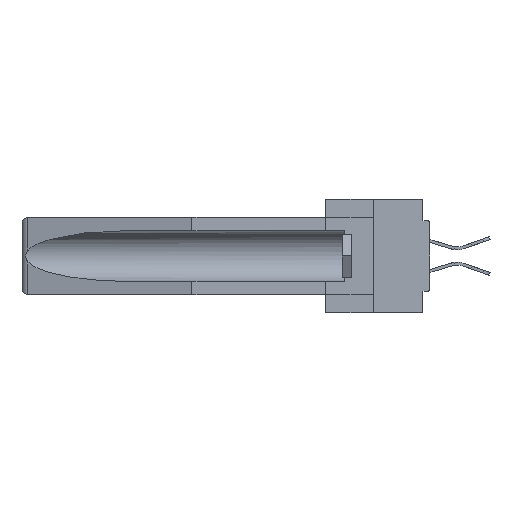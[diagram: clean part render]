
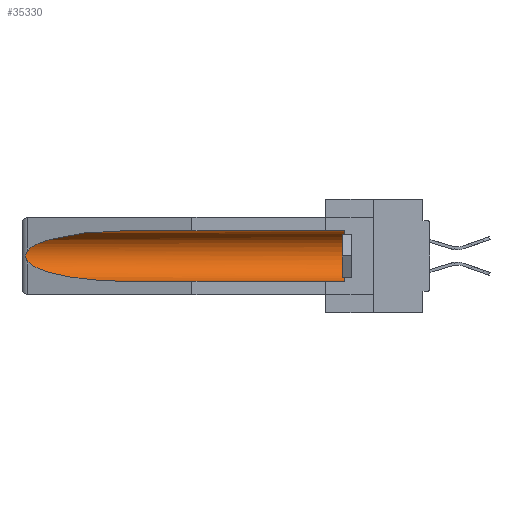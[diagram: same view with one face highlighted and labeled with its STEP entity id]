
A CAD part, left-side view. The second image highlights one B-rep face of the part: STEP entity #35330.
In plain terms, the highlighted cylindrical face has radius 2.857 mm (diameter 5.715 mm), a partial arc.
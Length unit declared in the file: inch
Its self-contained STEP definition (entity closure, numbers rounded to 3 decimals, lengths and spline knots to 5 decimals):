
#68 = DIRECTION ( 'NONE',  ( 0., 0., 1. ) ) ;
#99 = DIRECTION ( 'NONE',  ( 0., 0., 1. ) ) ;
#173 = CARTESIAN_POINT ( 'NONE',  ( 0.2673, 1.5327, -0.16383 ) ) ;
#321 = CARTESIAN_POINT ( 'NONE',  ( 0.2673, 1.53269, -0.17917 ) ) ;
#473 = CARTESIAN_POINT ( 'NONE',  ( 0.26654, 1.53092, -0.15636 ) ) ;
#629 = CARTESIAN_POINT ( 'NONE',  ( 0.26597, 1.5296, -0.19026 ) ) ;
#797 = LINE ( 'NONE', #43231, #3456 ) ;
#1778 = CARTESIAN_POINT ( 'NONE',  ( 0.26537, 1.52718, -0.19328 ) ) ;
#2358 = CARTESIAN_POINT ( 'NONE',  ( 0.21114, 1.30732, -0.284 ) ) ;
#3456 = VECTOR ( 'NONE', #29276, 39.37008 ) ;
#4014 = EDGE_CURVE ( 'NONE', #23667, #7533, #10403, .T. ) ;
#5608 = CARTESIAN_POINT ( 'NONE',  ( 0.155, 1.07973, -0.059 ) ) ;
#6609 = ORIENTED_EDGE ( 'NONE', *, *, #7077, .F. ) ;
#7077 = EDGE_CURVE ( 'NONE', #41100, #7533, #18135, .T. ) ;
#7160 = CARTESIAN_POINT ( 'NONE',  ( 0.26537, 1.52718, -0.19328 ) ) ;
#7533 = VERTEX_POINT ( 'NONE', #36277 ) ;
#10403 =( BOUNDED_CURVE ( )  B_SPLINE_CURVE ( 3, ( #1778, #12531, #2358, #19693 ),
 .UNSPECIFIED., .F., .F. ) 
 B_SPLINE_CURVE_WITH_KNOTS ( ( 4, 4 ),
 ( 0.1948, 1.5708 ),
 .UNSPECIFIED. ) 
 CURVE ( )  GEOMETRIC_REPRESENTATION_ITEM ( )  RATIONAL_B_SPLINE_CURVE ( ( 1., 0.848, 0.848, 1. ) ) 
 REPRESENTATION_ITEM ( '' )  );
#11840 = CARTESIAN_POINT ( 'NONE',  ( 0.155, 0.126, -0.059 ) ) ;
#12379 = ORIENTED_EDGE ( 'NONE', *, *, #4014, .T. ) ;
#12434 = CARTESIAN_POINT ( 'NONE',  ( 0.26537, 1.52718, -0.14972 ) ) ;
#12531 = CARTESIAN_POINT ( 'NONE',  ( 0.25451, 1.48313, -0.24835 ) ) ;
#13896 = DIRECTION ( 'NONE',  ( 0., -1., 0. ) ) ;
#13972 = CARTESIAN_POINT ( 'NONE',  ( 0.26537, 1.52718, -0.14972 ) ) ;
#13990 = CYLINDRICAL_SURFACE ( 'NONE', #24446, 0.1125 ) ;
#15562 = VERTEX_POINT ( 'NONE', #11840 ) ;
#15887 = VERTEX_POINT ( 'NONE', #28764 ) ;
#17029 = VECTOR ( 'NONE', #18907, 39.37008 ) ;
#17481 = CARTESIAN_POINT ( 'NONE',  ( 0.26597, 1.52961, -0.15275 ) ) ;
#17610 = ORIENTED_EDGE ( 'NONE', *, *, #39559, .T. ) ;
#17627 = CARTESIAN_POINT ( 'NONE',  ( 0.26655, 1.53094, -0.18657 ) ) ;
#18135 = LINE ( 'NONE', #43104, #17029 ) ;
#18243 = EDGE_CURVE ( 'NONE', #15887, #23667, #23204, .T. ) ;
#18907 = DIRECTION ( 'NONE',  ( 0., 1., 0. ) ) ;
#19693 = CARTESIAN_POINT ( 'NONE',  ( 0.155, 1.07973, -0.284 ) ) ;
#20891 = CARTESIAN_POINT ( 'NONE',  ( 0.155, 0.126, -0.1715 ) ) ;
#21831 = CARTESIAN_POINT ( 'NONE',  ( 0.26537, 1.52718, -0.19328 ) ) ;
#23025 = ORIENTED_EDGE ( 'NONE', *, *, #25254, .T. ) ;
#23195 = EDGE_LOOP ( 'NONE', ( #23025, #41322, #12379, #6609, #17610, #30607 ) ) ;
#23204 = B_SPLINE_CURVE_WITH_KNOTS ( 'NONE', 3,
 ( #13972, #17481, #473, #173, #24427, #24866, #321, #17627, #629, #7160 ),
 .UNSPECIFIED., .F., .F.,
 ( 4, 2, 2, 2, 4 ),
 ( 0., 0.00029, 0.00058, 0.00087, 0.00117 ),
 .UNSPECIFIED. ) ;
#23667 = VERTEX_POINT ( 'NONE', #21831 ) ;
#24427 = CARTESIAN_POINT ( 'NONE',  ( 0.2675, 1.53308, -0.16763 ) ) ;
#24446 = AXIS2_PLACEMENT_3D ( 'NONE', #31578, #38007, #68 ) ;
#24866 = CARTESIAN_POINT ( 'NONE',  ( 0.2675, 1.53308, -0.17534 ) ) ;
#25254 = EDGE_CURVE ( 'NONE', #31532, #15887, #38616, .T. ) ;
#27536 = CIRCLE ( 'NONE', #28947, 0.1125 ) ;
#28764 = CARTESIAN_POINT ( 'NONE',  ( 0.26537, 1.52718, -0.14972 ) ) ;
#28947 = AXIS2_PLACEMENT_3D ( 'NONE', #20891, #13896, #99 ) ;
#29276 = DIRECTION ( 'NONE',  ( 0., 1., 0. ) ) ;
#30150 = CARTESIAN_POINT ( 'NONE',  ( 0.25451, 1.48313, -0.09465 ) ) ;
#30607 = ORIENTED_EDGE ( 'NONE', *, *, #41426, .T. ) ;
#31532 = VERTEX_POINT ( 'NONE', #37404 ) ;
#31578 = CARTESIAN_POINT ( 'NONE',  ( 0.155, -0.30754, -0.1715 ) ) ;
#33619 = CARTESIAN_POINT ( 'NONE',  ( 0.21114, 1.30732, -0.059 ) ) ;
#34562 = FACE_OUTER_BOUND ( 'NONE', #23195, .T. ) ;
#35330 = ADVANCED_FACE ( 'NONE', ( #34562 ), #13990, .F. ) ;
#36277 = CARTESIAN_POINT ( 'NONE',  ( 0.155, 1.07973, -0.284 ) ) ;
#37404 = CARTESIAN_POINT ( 'NONE',  ( 0.155, 1.07973, -0.059 ) ) ;
#38007 = DIRECTION ( 'NONE',  ( 0., 1., 0. ) ) ;
#38616 =( BOUNDED_CURVE ( )  B_SPLINE_CURVE ( 3, ( #5608, #33619, #30150, #12434 ),
 .UNSPECIFIED., .F., .F. ) 
 B_SPLINE_CURVE_WITH_KNOTS ( ( 4, 4 ),
 ( 4.71239, 6.08839 ),
 .UNSPECIFIED. ) 
 CURVE ( )  GEOMETRIC_REPRESENTATION_ITEM ( )  RATIONAL_B_SPLINE_CURVE ( ( 1., 0.848, 0.848, 1. ) ) 
 REPRESENTATION_ITEM ( '' )  );
#39559 = EDGE_CURVE ( 'NONE', #41100, #15562, #27536, .T. ) ;
#41100 = VERTEX_POINT ( 'NONE', #41251 ) ;
#41251 = CARTESIAN_POINT ( 'NONE',  ( 0.155, 0.126, -0.284 ) ) ;
#41322 = ORIENTED_EDGE ( 'NONE', *, *, #18243, .T. ) ;
#41426 = EDGE_CURVE ( 'NONE', #15562, #31532, #797, .T. ) ;
#43104 = CARTESIAN_POINT ( 'NONE',  ( 0.155, -0.30754, -0.284 ) ) ;
#43231 = CARTESIAN_POINT ( 'NONE',  ( 0.155, -0.30754, -0.059 ) ) ;
